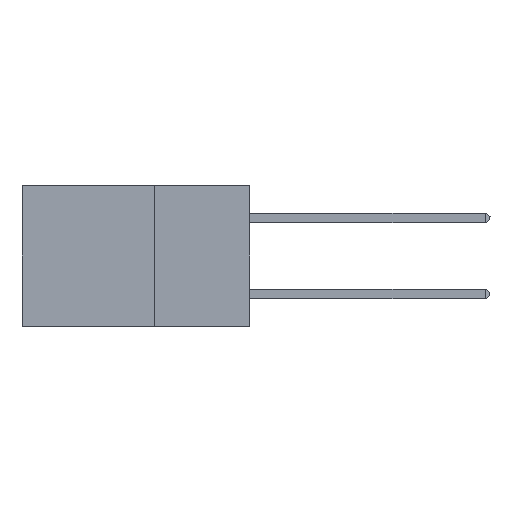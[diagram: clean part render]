
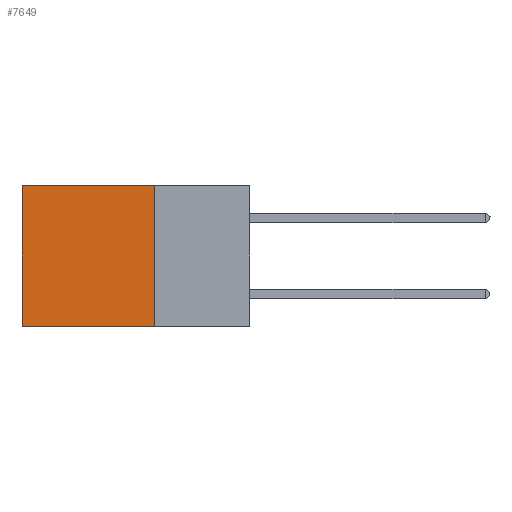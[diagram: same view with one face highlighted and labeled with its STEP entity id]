
A CAD part, left-side view. The second image highlights one B-rep face of the part: STEP entity #7649.
In plain terms, the highlighted planar face has unit normal (-1, 0, 0).
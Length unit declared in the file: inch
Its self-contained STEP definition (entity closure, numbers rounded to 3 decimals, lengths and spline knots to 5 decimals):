
#436 = ORIENTED_EDGE ( 'NONE', *, *, #28559, .F. ) ;
#909 = LINE ( 'NONE', #15089, #9043 ) ;
#1202 = CARTESIAN_POINT ( 'NONE',  ( 0.2875, 0.25, 0. ) ) ;
#1847 = CARTESIAN_POINT ( 'NONE',  ( 0.2875, 0.25, 0. ) ) ;
#2057 = DIRECTION ( 'NONE',  ( 0., 0., -1. ) ) ;
#7190 = VERTEX_POINT ( 'NONE', #8025 ) ;
#7649 = ADVANCED_FACE ( 'NONE', ( #32498 ), #29793, .F. ) ;
#7747 = EDGE_LOOP ( 'NONE', ( #26406, #436, #8155, #29629 ) ) ;
#8025 = CARTESIAN_POINT ( 'NONE',  ( 0.2875, 0.6, -0.37 ) ) ;
#8155 = ORIENTED_EDGE ( 'NONE', *, *, #29258, .F. ) ;
#9043 = VECTOR ( 'NONE', #27531, 39.37008 ) ;
#11431 = LINE ( 'NONE', #1847, #17295 ) ;
#12402 = CARTESIAN_POINT ( 'NONE',  ( 0.2875, 0.25, -0.37 ) ) ;
#14199 = VECTOR ( 'NONE', #15636, 39.37008 ) ;
#14231 = VERTEX_POINT ( 'NONE', #18351 ) ;
#15089 = CARTESIAN_POINT ( 'NONE',  ( 0.2875, 0.25, 0. ) ) ;
#15636 = DIRECTION ( 'NONE',  ( 0., 0., -1. ) ) ;
#16032 = VERTEX_POINT ( 'NONE', #30268 ) ;
#17052 = VERTEX_POINT ( 'NONE', #1202 ) ;
#17295 = VECTOR ( 'NONE', #24790, 39.37008 ) ;
#17438 = DIRECTION ( 'NONE',  ( 1., 0., 0. ) ) ;
#18351 = CARTESIAN_POINT ( 'NONE',  ( 0.2875, 0.25, -0.37 ) ) ;
#20485 = AXIS2_PLACEMENT_3D ( 'NONE', #32383, #17438, #2057 ) ;
#21039 = VECTOR ( 'NONE', #27348, 39.37008 ) ;
#24609 = EDGE_CURVE ( 'NONE', #16032, #7190, #27487, .T. ) ;
#24790 = DIRECTION ( 'NONE',  ( 0., 1., 0. ) ) ;
#26406 = ORIENTED_EDGE ( 'NONE', *, *, #24609, .T. ) ;
#27348 = DIRECTION ( 'NONE',  ( 0., 1., 0. ) ) ;
#27487 = LINE ( 'NONE', #28102, #14199 ) ;
#27531 = DIRECTION ( 'NONE',  ( 0., 0., -1. ) ) ;
#27661 = LINE ( 'NONE', #12402, #21039 ) ;
#28102 = CARTESIAN_POINT ( 'NONE',  ( 0.2875, 0.6, 0. ) ) ;
#28559 = EDGE_CURVE ( 'NONE', #14231, #7190, #27661, .T. ) ;
#29258 = EDGE_CURVE ( 'NONE', #17052, #14231, #909, .T. ) ;
#29629 = ORIENTED_EDGE ( 'NONE', *, *, #30156, .T. ) ;
#29793 = PLANE ( 'NONE',  #20485 ) ;
#30156 = EDGE_CURVE ( 'NONE', #17052, #16032, #11431, .T. ) ;
#30268 = CARTESIAN_POINT ( 'NONE',  ( 0.2875, 0.6, 0. ) ) ;
#32383 = CARTESIAN_POINT ( 'NONE',  ( 0.2875, 0.25, 0. ) ) ;
#32498 = FACE_OUTER_BOUND ( 'NONE', #7747, .T. ) ;
